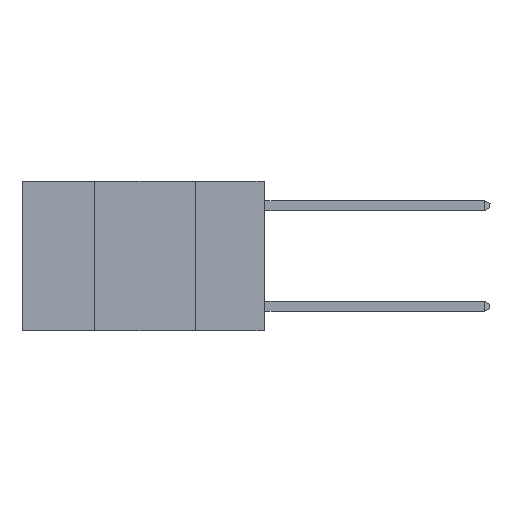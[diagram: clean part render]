
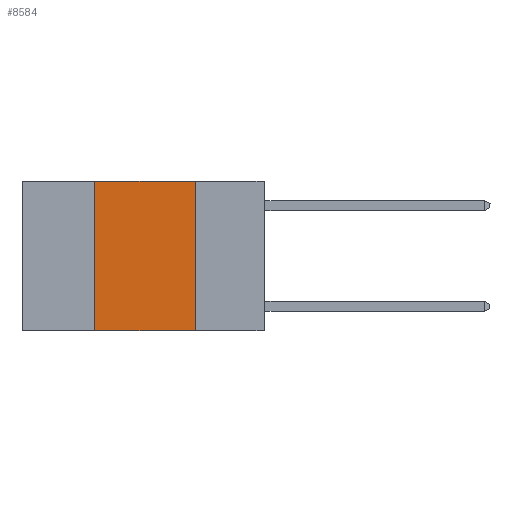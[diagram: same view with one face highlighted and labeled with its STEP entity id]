
A CAD part, left-side view. The second image highlights one B-rep face of the part: STEP entity #8584.
In plain terms, the highlighted planar face has unit normal (-1, 0, 0).
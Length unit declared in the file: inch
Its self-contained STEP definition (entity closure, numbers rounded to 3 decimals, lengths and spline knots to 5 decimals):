
#41 = CARTESIAN_POINT ( 'NONE',  ( 0., 0.42, 0. ) ) ;
#193 = VECTOR ( 'NONE', #4199, 39.37008 ) ;
#907 = VERTEX_POINT ( 'NONE', #5904 ) ;
#948 = DIRECTION ( 'NONE',  ( 1., 0., 0. ) ) ;
#1732 = LINE ( 'NONE', #12934, #6053 ) ;
#2044 = DIRECTION ( 'NONE',  ( 0., 0., -1. ) ) ;
#2376 = LINE ( 'NONE', #5622, #4841 ) ;
#3568 = DIRECTION ( 'NONE',  ( 0., 0., 1. ) ) ;
#4143 = EDGE_CURVE ( 'NONE', #5201, #907, #1732, .T. ) ;
#4177 = ORIENTED_EDGE ( 'NONE', *, *, #11664, .F. ) ;
#4199 = DIRECTION ( 'NONE',  ( 0., -1., 0. ) ) ;
#4326 = LINE ( 'NONE', #7331, #193 ) ;
#4508 = VERTEX_POINT ( 'NONE', #11361 ) ;
#4719 = ORIENTED_EDGE ( 'NONE', *, *, #4143, .T. ) ;
#4841 = VECTOR ( 'NONE', #3568, 39.37008 ) ;
#5201 = VERTEX_POINT ( 'NONE', #5373 ) ;
#5373 = CARTESIAN_POINT ( 'NONE',  ( 0., 0.42, -0.37 ) ) ;
#5622 = CARTESIAN_POINT ( 'NONE',  ( 0., 0.42, 0. ) ) ;
#5641 = ORIENTED_EDGE ( 'NONE', *, *, #13142, .F. ) ;
#5904 = CARTESIAN_POINT ( 'NONE',  ( 0., 0.17, -0.37 ) ) ;
#6053 = VECTOR ( 'NONE', #10254, 39.37008 ) ;
#6745 = VECTOR ( 'NONE', #2044, 39.37008 ) ;
#6772 = AXIS2_PLACEMENT_3D ( 'NONE', #7334, #948, #9302 ) ;
#7331 = CARTESIAN_POINT ( 'NONE',  ( 0., 0.6, 0. ) ) ;
#7334 = CARTESIAN_POINT ( 'NONE',  ( 0., 0.6, 0. ) ) ;
#7541 = CARTESIAN_POINT ( 'NONE',  ( 0., 0.17, 0. ) ) ;
#8584 = ADVANCED_FACE ( 'NONE', ( #11792 ), #10322, .F. ) ;
#9212 = ORIENTED_EDGE ( 'NONE', *, *, #13299, .F. ) ;
#9302 = DIRECTION ( 'NONE',  ( 0., 0., -1. ) ) ;
#9609 = VERTEX_POINT ( 'NONE', #41 ) ;
#10254 = DIRECTION ( 'NONE',  ( 0., -1., 0. ) ) ;
#10322 = PLANE ( 'NONE',  #6772 ) ;
#10416 = EDGE_LOOP ( 'NONE', ( #4177, #5641, #9212, #4719 ) ) ;
#11361 = CARTESIAN_POINT ( 'NONE',  ( 0., 0.17, 0. ) ) ;
#11664 = EDGE_CURVE ( 'NONE', #4508, #907, #12720, .T. ) ;
#11792 = FACE_OUTER_BOUND ( 'NONE', #10416, .T. ) ;
#12720 = LINE ( 'NONE', #7541, #6745 ) ;
#12934 = CARTESIAN_POINT ( 'NONE',  ( 0., 0.6, -0.37 ) ) ;
#13142 = EDGE_CURVE ( 'NONE', #9609, #4508, #4326, .T. ) ;
#13299 = EDGE_CURVE ( 'NONE', #5201, #9609, #2376, .T. ) ;
